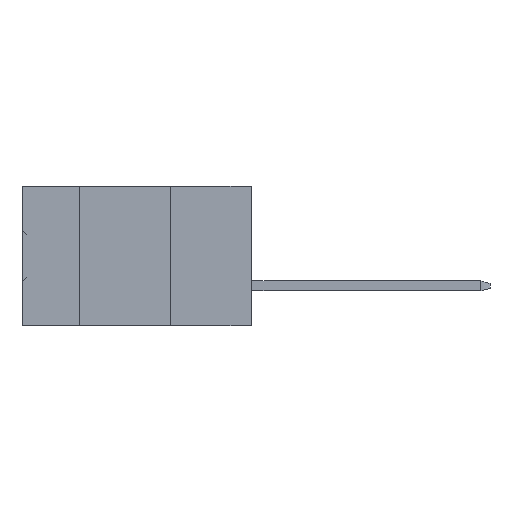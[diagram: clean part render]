
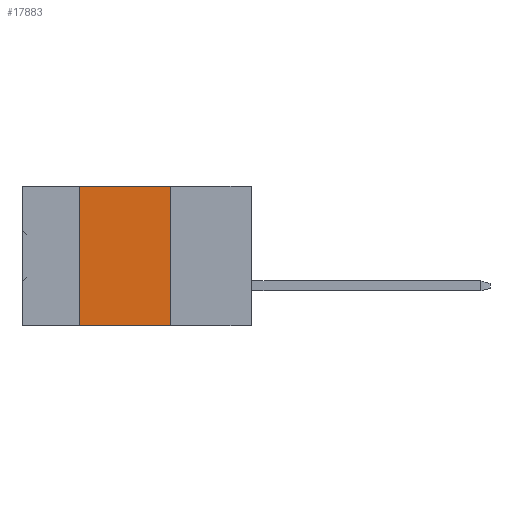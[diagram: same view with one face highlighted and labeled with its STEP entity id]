
A CAD part, left-side view. The second image highlights one B-rep face of the part: STEP entity #17883.
In plain terms, the highlighted planar face has unit normal (-1, 0, 0).
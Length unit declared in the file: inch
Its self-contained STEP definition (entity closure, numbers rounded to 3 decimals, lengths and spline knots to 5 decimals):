
#2835 = LINE ( 'NONE', #12197, #13488 ) ;
#3604 = EDGE_CURVE ( 'NONE', #15747, #19983, #2835, .T. ) ;
#3925 = CARTESIAN_POINT ( 'NONE',  ( 0., 0.254, -0.437 ) ) ;
#4007 = VECTOR ( 'NONE', #29886, 39.37008 ) ;
#4342 = VERTEX_POINT ( 'NONE', #18039 ) ;
#5094 = CARTESIAN_POINT ( 'NONE',  ( 0., 0.72, 0. ) ) ;
#7399 = PLANE ( 'NONE',  #30478 ) ;
#7744 = CARTESIAN_POINT ( 'NONE',  ( 0., 0.54, 0. ) ) ;
#8131 = LINE ( 'NONE', #22609, #23281 ) ;
#9399 = FACE_OUTER_BOUND ( 'NONE', #9655, .T. ) ;
#9655 = EDGE_LOOP ( 'NONE', ( #9737, #27605, #11682, #24415 ) ) ;
#9737 = ORIENTED_EDGE ( 'NONE', *, *, #11229, .F. ) ;
#11073 = LINE ( 'NONE', #23091, #4007 ) ;
#11229 = EDGE_CURVE ( 'NONE', #4342, #19983, #20090, .T. ) ;
#11682 = ORIENTED_EDGE ( 'NONE', *, *, #19747, .F. ) ;
#11856 = DIRECTION ( 'NONE',  ( 1., 0., 0. ) ) ;
#11921 = CARTESIAN_POINT ( 'NONE',  ( 0., 0.54, -0.437 ) ) ;
#12197 = CARTESIAN_POINT ( 'NONE',  ( 0., 0.72, -0.437 ) ) ;
#13453 = DIRECTION ( 'NONE',  ( 0., 0., -1. ) ) ;
#13488 = VECTOR ( 'NONE', #28723, 39.37008 ) ;
#13540 = VECTOR ( 'NONE', #13453, 39.37008 ) ;
#15747 = VERTEX_POINT ( 'NONE', #11921 ) ;
#17883 = ADVANCED_FACE ( 'NONE', ( #9399 ), #7399, .F. ) ;
#18039 = CARTESIAN_POINT ( 'NONE',  ( 0., 0.254, 0. ) ) ;
#19747 = EDGE_CURVE ( 'NONE', #15747, #22098, #11073, .T. ) ;
#19983 = VERTEX_POINT ( 'NONE', #21223 ) ;
#20090 = LINE ( 'NONE', #3925, #13540 ) ;
#21223 = CARTESIAN_POINT ( 'NONE',  ( 0., 0.254, -0.437 ) ) ;
#21256 = DIRECTION ( 'NONE',  ( 0., 0., -1. ) ) ;
#22098 = VERTEX_POINT ( 'NONE', #7744 ) ;
#22141 = DIRECTION ( 'NONE',  ( 0., -1., 0. ) ) ;
#22609 = CARTESIAN_POINT ( 'NONE',  ( 0., 0.72, 0. ) ) ;
#22695 = EDGE_CURVE ( 'NONE', #22098, #4342, #8131, .T. ) ;
#23091 = CARTESIAN_POINT ( 'NONE',  ( 0., 0.54, -0.437 ) ) ;
#23281 = VECTOR ( 'NONE', #22141, 39.37008 ) ;
#24415 = ORIENTED_EDGE ( 'NONE', *, *, #3604, .T. ) ;
#27605 = ORIENTED_EDGE ( 'NONE', *, *, #22695, .F. ) ;
#28723 = DIRECTION ( 'NONE',  ( 0., -1., 0. ) ) ;
#29886 = DIRECTION ( 'NONE',  ( 0., 0., 1. ) ) ;
#30478 = AXIS2_PLACEMENT_3D ( 'NONE', #5094, #11856, #21256 ) ;
